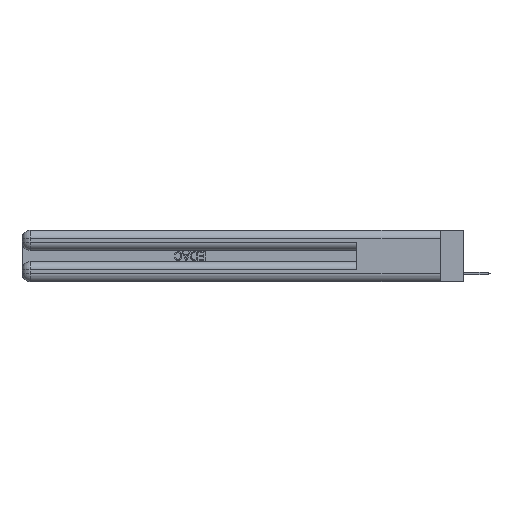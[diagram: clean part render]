
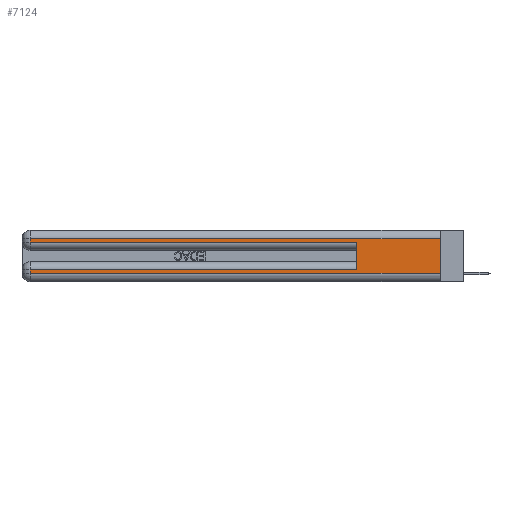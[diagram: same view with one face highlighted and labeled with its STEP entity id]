
A CAD part, left-side view. The second image highlights one B-rep face of the part: STEP entity #7124.
In plain terms, the highlighted planar face has unit normal (-1, 0, 0).
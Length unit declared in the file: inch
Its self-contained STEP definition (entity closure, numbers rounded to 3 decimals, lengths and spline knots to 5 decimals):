
#1742 = CARTESIAN_POINT ( 'NONE',  ( 0., 2.94, 0.37 ) ) ;
#3223 = LINE ( 'NONE', #20459, #12683 ) ;
#3260 = DIRECTION ( 'NONE',  ( 0., -1., 0. ) ) ;
#4313 = VERTEX_POINT ( 'NONE', #22088 ) ;
#4694 = FACE_OUTER_BOUND ( 'NONE', #21241, .T. ) ;
#4932 = ORIENTED_EDGE ( 'NONE', *, *, #17813, .T. ) ;
#4977 = VECTOR ( 'NONE', #3260, 39.37008 ) ;
#5192 = DIRECTION ( 'NONE',  ( 1., 0., 0. ) ) ;
#5286 = VECTOR ( 'NONE', #29798, 39.37008 ) ;
#5398 = LINE ( 'NONE', #1742, #11303 ) ;
#5656 = DIRECTION ( 'NONE',  ( 0., 0., -1. ) ) ;
#6048 = EDGE_CURVE ( 'NONE', #27783, #21664, #3223, .T. ) ;
#6170 = CARTESIAN_POINT ( 'NONE',  ( 0., 2.94, 0.06 ) ) ;
#7124 = ADVANCED_FACE ( 'NONE', ( #4694 ), #27808, .F. ) ;
#7975 = CARTESIAN_POINT ( 'NONE',  ( 0., 0., 0.37 ) ) ;
#8112 = CARTESIAN_POINT ( 'NONE',  ( 0., 0.6, 0.285 ) ) ;
#8619 = EDGE_CURVE ( 'NONE', #4313, #25716, #5398, .T. ) ;
#8731 = CARTESIAN_POINT ( 'NONE',  ( 0., 0., 0.31 ) ) ;
#8997 = CARTESIAN_POINT ( 'NONE',  ( 0., 0., 0.285 ) ) ;
#9437 = CARTESIAN_POINT ( 'NONE',  ( 0., 0., 0.06 ) ) ;
#10364 = VERTEX_POINT ( 'NONE', #8112 ) ;
#10501 = CARTESIAN_POINT ( 'NONE',  ( 0., 0., 0.085 ) ) ;
#10598 = DIRECTION ( 'NONE',  ( 0., 0., -1. ) ) ;
#11273 = ORIENTED_EDGE ( 'NONE', *, *, #25541, .T. ) ;
#11303 = VECTOR ( 'NONE', #14636, 39.37008 ) ;
#11715 = EDGE_CURVE ( 'NONE', #26809, #29297, #11938, .T. ) ;
#11938 = LINE ( 'NONE', #10501, #22880 ) ;
#12683 = VECTOR ( 'NONE', #10598, 39.37008 ) ;
#12791 = CARTESIAN_POINT ( 'NONE',  ( 0., 0.6, 0.085 ) ) ;
#14636 = DIRECTION ( 'NONE',  ( 0., 0., -1. ) ) ;
#15366 = ORIENTED_EDGE ( 'NONE', *, *, #6048, .F. ) ;
#15865 = LINE ( 'NONE', #31531, #25586 ) ;
#16596 = EDGE_CURVE ( 'NONE', #30919, #21664, #18640, .T. ) ;
#17579 = LINE ( 'NONE', #25436, #19101 ) ;
#17636 = DIRECTION ( 'NONE',  ( 0., 1., 0. ) ) ;
#17813 = EDGE_CURVE ( 'NONE', #27783, #4313, #28541, .T. ) ;
#18338 = LINE ( 'NONE', #8997, #4977 ) ;
#18422 = ORIENTED_EDGE ( 'NONE', *, *, #21094, .F. ) ;
#18640 = LINE ( 'NONE', #32222, #5286 ) ;
#19101 = VECTOR ( 'NONE', #5656, 39.37008 ) ;
#19183 = ORIENTED_EDGE ( 'NONE', *, *, #16596, .T. ) ;
#19332 = CARTESIAN_POINT ( 'NONE',  ( 0., 2.94, 0.085 ) ) ;
#20414 = VECTOR ( 'NONE', #24119, 39.37008 ) ;
#20459 = CARTESIAN_POINT ( 'NONE',  ( 0., 0., 0.37 ) ) ;
#21094 = EDGE_CURVE ( 'NONE', #26809, #10364, #15865, .T. ) ;
#21241 = EDGE_LOOP ( 'NONE', ( #15366, #4932, #27160, #11273, #18422, #25457, #25531, #19183 ) ) ;
#21664 = VERTEX_POINT ( 'NONE', #9437 ) ;
#21986 = CARTESIAN_POINT ( 'NONE',  ( 0., 0., 0.31 ) ) ;
#22088 = CARTESIAN_POINT ( 'NONE',  ( 0., 2.94, 0.31 ) ) ;
#22880 = VECTOR ( 'NONE', #17636, 39.37008 ) ;
#24119 = DIRECTION ( 'NONE',  ( 0., 1., 0. ) ) ;
#25436 = CARTESIAN_POINT ( 'NONE',  ( 0., 2.94, 0.37 ) ) ;
#25457 = ORIENTED_EDGE ( 'NONE', *, *, #11715, .T. ) ;
#25531 = ORIENTED_EDGE ( 'NONE', *, *, #26220, .T. ) ;
#25541 = EDGE_CURVE ( 'NONE', #25716, #10364, #18338, .T. ) ;
#25586 = VECTOR ( 'NONE', #26661, 39.37008 ) ;
#25716 = VERTEX_POINT ( 'NONE', #30296 ) ;
#26220 = EDGE_CURVE ( 'NONE', #29297, #30919, #17579, .T. ) ;
#26661 = DIRECTION ( 'NONE',  ( 0., 0., 1. ) ) ;
#26809 = VERTEX_POINT ( 'NONE', #12791 ) ;
#27160 = ORIENTED_EDGE ( 'NONE', *, *, #8619, .T. ) ;
#27783 = VERTEX_POINT ( 'NONE', #21986 ) ;
#27808 = PLANE ( 'NONE',  #32343 ) ;
#28541 = LINE ( 'NONE', #8731, #20414 ) ;
#29297 = VERTEX_POINT ( 'NONE', #19332 ) ;
#29798 = DIRECTION ( 'NONE',  ( 0., -1., 0. ) ) ;
#29969 = DIRECTION ( 'NONE',  ( 0., 0., -1. ) ) ;
#30296 = CARTESIAN_POINT ( 'NONE',  ( 0., 2.94, 0.285 ) ) ;
#30919 = VERTEX_POINT ( 'NONE', #6170 ) ;
#31531 = CARTESIAN_POINT ( 'NONE',  ( 0., 0.6, 0.145 ) ) ;
#32222 = CARTESIAN_POINT ( 'NONE',  ( 0., 0., 0.06 ) ) ;
#32343 = AXIS2_PLACEMENT_3D ( 'NONE', #7975, #5192, #29969 ) ;
